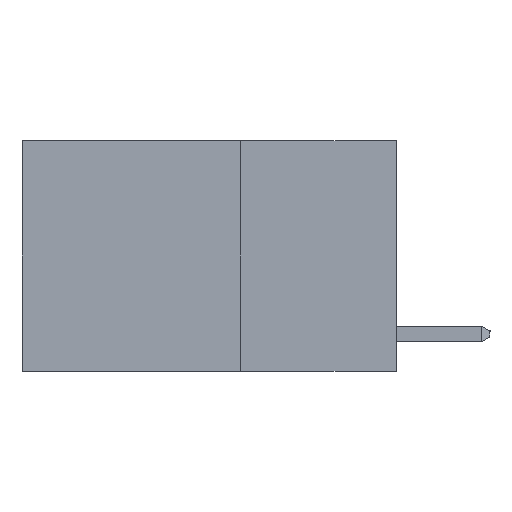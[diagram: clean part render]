
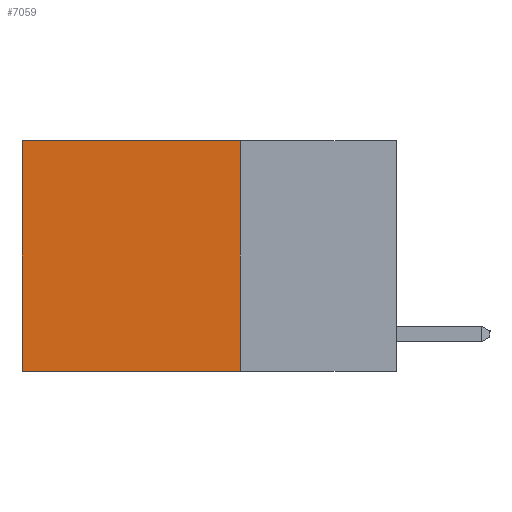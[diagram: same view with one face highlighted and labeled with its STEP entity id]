
A CAD part, left-side view. The second image highlights one B-rep face of the part: STEP entity #7059.
In plain terms, the highlighted planar face has unit normal (-1, 0, 0).
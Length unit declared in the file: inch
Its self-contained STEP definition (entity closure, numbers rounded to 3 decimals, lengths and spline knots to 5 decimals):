
#135 = CARTESIAN_POINT ( 'NONE',  ( 0.2625, 0.25, 0. ) ) ;
#581 = ORIENTED_EDGE ( 'NONE', *, *, #8993, .T. ) ;
#840 = CARTESIAN_POINT ( 'NONE',  ( 0.2625, 0.25, -0.37 ) ) ;
#1031 = ORIENTED_EDGE ( 'NONE', *, *, #5564, .T. ) ;
#1561 = DIRECTION ( 'NONE',  ( 0., 0., -1. ) ) ;
#1754 = CARTESIAN_POINT ( 'NONE',  ( 0.2625, 0.25, 0. ) ) ;
#2009 = LINE ( 'NONE', #4857, #5449 ) ;
#2919 = AXIS2_PLACEMENT_3D ( 'NONE', #1754, #10711, #3130 ) ;
#3130 = DIRECTION ( 'NONE',  ( 0., 0., -1. ) ) ;
#3570 = EDGE_LOOP ( 'NONE', ( #581, #7448, #14130, #1031 ) ) ;
#3604 = FACE_OUTER_BOUND ( 'NONE', #3570, .T. ) ;
#3856 = CARTESIAN_POINT ( 'NONE',  ( 0.2625, 0.25, 0. ) ) ;
#4335 = CARTESIAN_POINT ( 'NONE',  ( 0.2625, 0.6, -0.37 ) ) ;
#4818 = VERTEX_POINT ( 'NONE', #4335 ) ;
#4857 = CARTESIAN_POINT ( 'NONE',  ( 0.2625, 0.25, -0.37 ) ) ;
#5023 = CARTESIAN_POINT ( 'NONE',  ( 0.2625, 0.25, 0. ) ) ;
#5089 = DIRECTION ( 'NONE',  ( 0., 1., 0. ) ) ;
#5449 = VECTOR ( 'NONE', #12406, 39.37008 ) ;
#5564 = EDGE_CURVE ( 'NONE', #16332, #14538, #5607, .T. ) ;
#5607 = LINE ( 'NONE', #3856, #11928 ) ;
#6457 = VECTOR ( 'NONE', #11262, 39.37008 ) ;
#7059 = ADVANCED_FACE ( 'NONE', ( #3604 ), #9444, .F. ) ;
#7448 = ORIENTED_EDGE ( 'NONE', *, *, #9986, .F. ) ;
#8285 = EDGE_CURVE ( 'NONE', #16332, #12021, #16339, .T. ) ;
#8993 = EDGE_CURVE ( 'NONE', #14538, #4818, #10257, .T. ) ;
#9444 = PLANE ( 'NONE',  #2919 ) ;
#9986 = EDGE_CURVE ( 'NONE', #12021, #4818, #2009, .T. ) ;
#10257 = LINE ( 'NONE', #12492, #6457 ) ;
#10711 = DIRECTION ( 'NONE',  ( 1., 0., 0. ) ) ;
#11262 = DIRECTION ( 'NONE',  ( 0., 0., -1. ) ) ;
#11657 = CARTESIAN_POINT ( 'NONE',  ( 0.2625, 0.6, 0. ) ) ;
#11928 = VECTOR ( 'NONE', #5089, 39.37008 ) ;
#12021 = VERTEX_POINT ( 'NONE', #840 ) ;
#12406 = DIRECTION ( 'NONE',  ( 0., 1., 0. ) ) ;
#12492 = CARTESIAN_POINT ( 'NONE',  ( 0.2625, 0.6, 0. ) ) ;
#14130 = ORIENTED_EDGE ( 'NONE', *, *, #8285, .F. ) ;
#14538 = VERTEX_POINT ( 'NONE', #11657 ) ;
#15235 = VECTOR ( 'NONE', #1561, 39.37008 ) ;
#16332 = VERTEX_POINT ( 'NONE', #5023 ) ;
#16339 = LINE ( 'NONE', #135, #15235 ) ;
